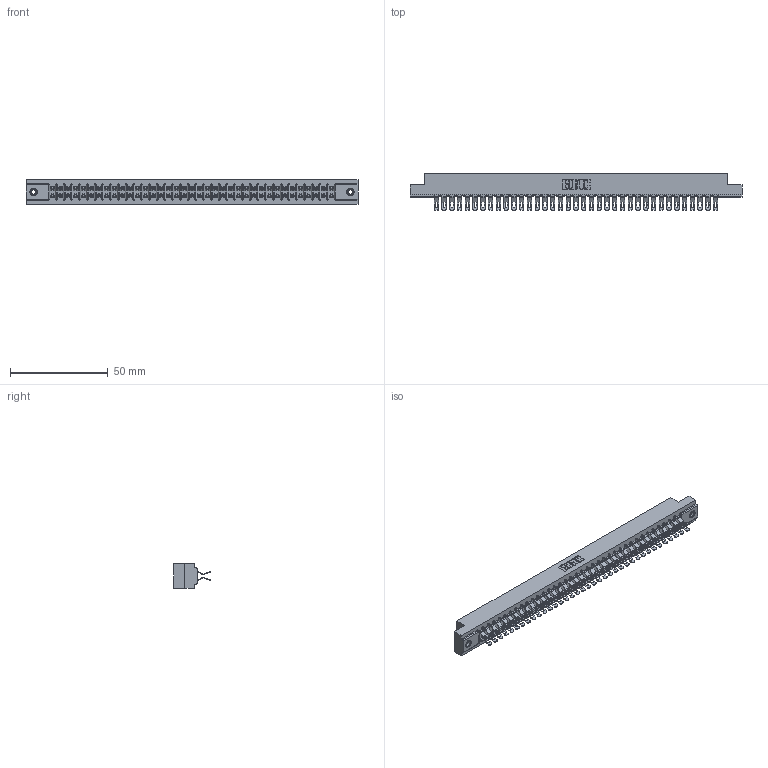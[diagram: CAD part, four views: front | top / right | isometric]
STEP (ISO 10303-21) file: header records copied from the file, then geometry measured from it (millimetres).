
FILE_DESCRIPTION (( 'STEP AP203' ), '1' );
FILE_NAME ('307-074-555-208.STEP', '2019-09-06T21:18:54', ( '' ), ( '' ), 'SwSTEP 2.0', 'SolidWorks 2016', '' );
FILE_SCHEMA (( 'CONFIG_CONTROL_DESIGN' ));
Length unit declared in the file: inch
Products named in the file (4): 307-290-001_555; 345-250-001_345-250-003-102; 307-074-555-208; 307 Part_.156 Dia Mounting Holes
Assembly tree (77 placements, depth 2):
  307-074-555-208
    307 Part_.156 Dia Mounting Holes
    307-290-001_555  x74
    345-250-001_345-250-003-102  x2
Bounding box: 169.62 x 18.75 x 12.7 mm (x, y, z)
Volume: 18215.7 mm3; surface area: 23431.4 mm2
Topology: 77 solids, 77 shells, 4730 faces, 13853 edges, 9026 vertices
Faces by surface type: plane 2618, cylinder 2020, sphere 76, cone 12, torus 4
Entity records: 35242 total; most frequent: CARTESIAN_POINT 5756, ORIENTED_EDGE 5700, DIRECTION 5656, EDGE_CURVE 2850, LINE 2172, VECTOR 2172, VERTEX_POINT 1842, AXIS2_PLACEMENT_3D 1742
